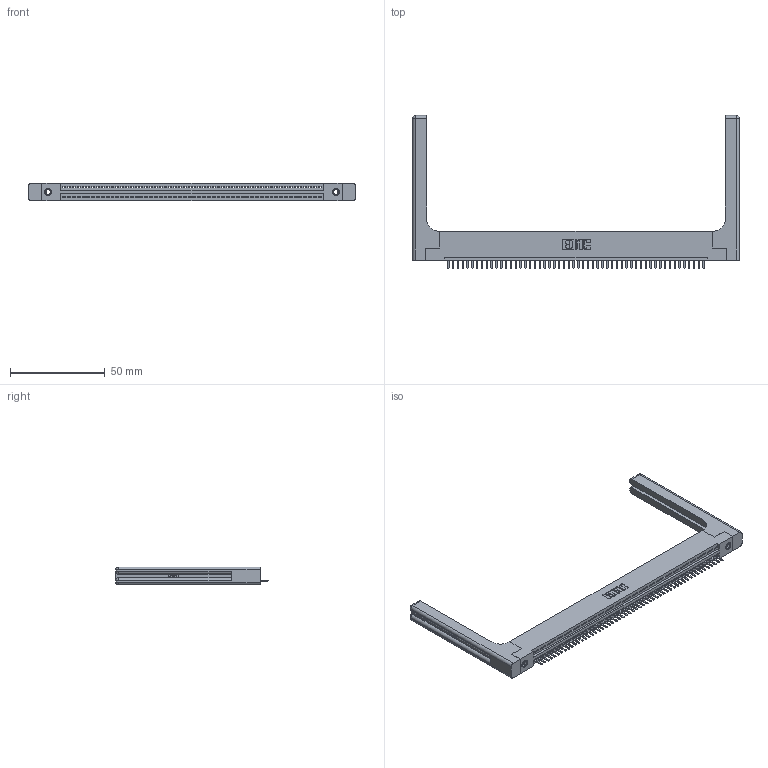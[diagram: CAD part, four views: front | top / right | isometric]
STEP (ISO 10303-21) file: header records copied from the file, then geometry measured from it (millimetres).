
FILE_DESCRIPTION (( 'STEP AP203' ), '1' );
FILE_NAME ('345-054-520-158.STEP', '2019-10-09T22:41:30', ( '' ), ( '' ), 'SwSTEP 2.0', 'SolidWorks 2016', '' );
FILE_SCHEMA (( 'CONFIG_CONTROL_DESIGN' ));
Length unit declared in the file: inch
Products named in the file (5): 345-054-520-158; 345-220-058_345-220-058; 345 Part_Flush Mounting Lugs - 0.156 Dia-TH; 345-292-001_345-293-120; 345-250-001_345-250-001-102
Assembly tree (59 placements, depth 2):
  345-054-520-158
    345 Part_Flush Mounting Lugs - 0.156 Dia-TH
    345-292-001_345-293-120  x54
    345-250-001_345-250-001-102  x2
    345-220-058_345-220-058  x2
Bounding box: 172.19 x 80.64 x 9.4 mm (x, y, z)
Volume: 24802.4 mm3; surface area: 26618.3 mm2
Topology: 59 solids, 59 shells, 3730 faces, 10943 edges, 7130 vertices
Faces by surface type: plane 2496, cylinder 1174, bspline 36, cone 12, sphere 8, torus 4
Entity records: 44322 total; most frequent: CARTESIAN_POINT 8659, ORIENTED_EDGE 7432, DIRECTION 6480, EDGE_CURVE 3716, VECTOR 3272, LINE 3272, VERTEX_POINT 2466, AXIS2_PLACEMENT_3D 1604
